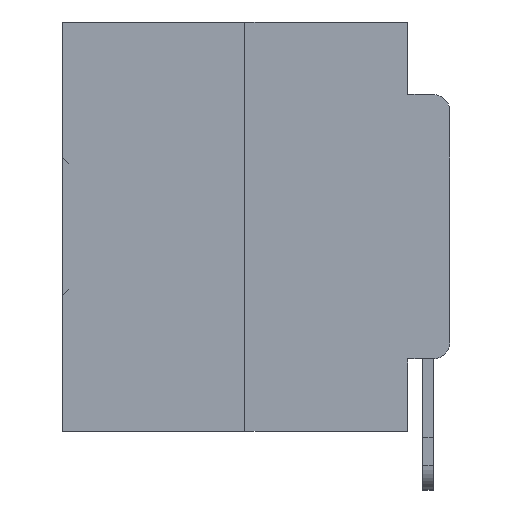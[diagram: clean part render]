
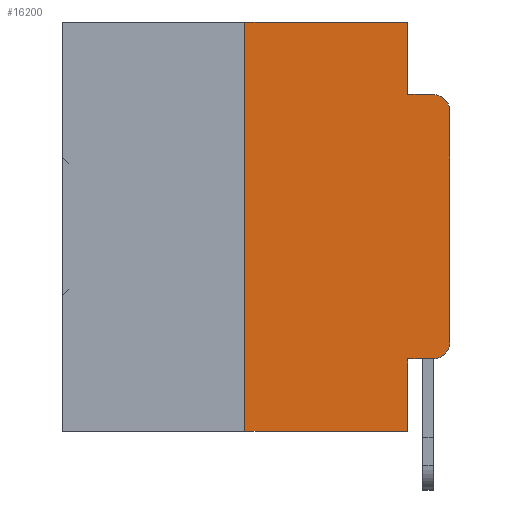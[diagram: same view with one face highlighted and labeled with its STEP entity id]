
A CAD part, left-side view. The second image highlights one B-rep face of the part: STEP entity #16200.
In plain terms, the highlighted planar face has unit normal (-1, 0, 0).
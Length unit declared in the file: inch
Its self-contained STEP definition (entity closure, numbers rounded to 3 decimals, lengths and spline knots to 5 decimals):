
#316 = ORIENTED_EDGE ( 'NONE', *, *, #16599, .T. ) ;
#415 = LINE ( 'NONE', #3776, #14605 ) ;
#475 = CARTESIAN_POINT ( 'NONE',  ( 0., 0.02, -0.1085 ) ) ;
#626 = AXIS2_PLACEMENT_3D ( 'NONE', #31320, #15009, #33985 ) ;
#838 = ORIENTED_EDGE ( 'NONE', *, *, #1508, .T. ) ;
#1125 = ORIENTED_EDGE ( 'NONE', *, *, #10313, .T. ) ;
#1165 = ORIENTED_EDGE ( 'NONE', *, *, #22442, .F. ) ;
#1508 = EDGE_CURVE ( 'NONE', #34756, #16977, #32853, .T. ) ;
#1520 = CARTESIAN_POINT ( 'NONE',  ( 0., 0.051, -0.4115 ) ) ;
#2182 = DIRECTION ( 'NONE',  ( 0., 0., -1. ) ) ;
#2471 = EDGE_CURVE ( 'NONE', #23822, #13464, #30337, .T. ) ;
#2742 = ORIENTED_EDGE ( 'NONE', *, *, #3702, .F. ) ;
#2930 = CARTESIAN_POINT ( 'NONE',  ( 0., 0.051, -0.4115 ) ) ;
#3365 = DIRECTION ( 'NONE',  ( 0., 0., -1. ) ) ;
#3394 = VERTEX_POINT ( 'NONE', #32758 ) ;
#3702 = EDGE_CURVE ( 'NONE', #13464, #31263, #34383, .T. ) ;
#3776 = CARTESIAN_POINT ( 'NONE',  ( 0., 0.051, 0. ) ) ;
#4247 = VECTOR ( 'NONE', #34108, 39.37008 ) ;
#5281 = EDGE_LOOP ( 'NONE', ( #1125, #838, #5604, #1165, #2742, #10926, #316, #14010, #35750, #34200 ) ) ;
#5604 = ORIENTED_EDGE ( 'NONE', *, *, #24743, .F. ) ;
#5786 = EDGE_CURVE ( 'NONE', #6816, #3394, #32164, .T. ) ;
#6456 = LINE ( 'NONE', #19384, #34750 ) ;
#6816 = VERTEX_POINT ( 'NONE', #9810 ) ;
#7062 = VECTOR ( 'NONE', #35310, 39.37008 ) ;
#7760 = CARTESIAN_POINT ( 'NONE',  ( 0., 0.051, 0. ) ) ;
#8363 = VECTOR ( 'NONE', #26809, 39.37008 ) ;
#8773 = LINE ( 'NONE', #1520, #22715 ) ;
#8868 = DIRECTION ( 'NONE',  ( 0., -1., 0. ) ) ;
#9810 = CARTESIAN_POINT ( 'NONE',  ( 0., 0.02, -0.4115 ) ) ;
#10313 = EDGE_CURVE ( 'NONE', #3394, #34756, #6456, .T. ) ;
#10926 = ORIENTED_EDGE ( 'NONE', *, *, #2471, .F. ) ;
#11040 = DIRECTION ( 'NONE',  ( 0., 0., 1. ) ) ;
#11996 = CARTESIAN_POINT ( 'NONE',  ( 0., 0., -0.1085 ) ) ;
#12901 = CARTESIAN_POINT ( 'NONE',  ( 0., 0.25, -0.5 ) ) ;
#13464 = VERTEX_POINT ( 'NONE', #29879 ) ;
#13774 = CARTESIAN_POINT ( 'NONE',  ( 0., 0.051, -0.5 ) ) ;
#14010 = ORIENTED_EDGE ( 'NONE', *, *, #14531, .F. ) ;
#14379 = VECTOR ( 'NONE', #8868, 39.37008 ) ;
#14531 = EDGE_CURVE ( 'NONE', #31238, #26175, #24023, .T. ) ;
#14605 = VECTOR ( 'NONE', #23334, 39.37008 ) ;
#15009 = DIRECTION ( 'NONE',  ( 1., 0., 0. ) ) ;
#15206 = EDGE_CURVE ( 'NONE', #31238, #6816, #8773, .T. ) ;
#15773 = CARTESIAN_POINT ( 'NONE',  ( 0., 0.25, 0. ) ) ;
#16200 = ADVANCED_FACE ( 'NONE', ( #27295 ), #33211, .F. ) ;
#16424 = CARTESIAN_POINT ( 'NONE',  ( 0., 0.051, -0.0885 ) ) ;
#16599 = EDGE_CURVE ( 'NONE', #23822, #26175, #21743, .T. ) ;
#16977 = VERTEX_POINT ( 'NONE', #21761 ) ;
#19093 = DIRECTION ( 'NONE',  ( -1., 0., 0. ) ) ;
#19384 = CARTESIAN_POINT ( 'NONE',  ( 0., 0., 0. ) ) ;
#19810 = VERTEX_POINT ( 'NONE', #34322 ) ;
#20209 = DIRECTION ( 'NONE',  ( -1., 0., 0. ) ) ;
#21052 = LINE ( 'NONE', #16424, #7062 ) ;
#21675 = DIRECTION ( 'NONE',  ( 0., 0., -1. ) ) ;
#21743 = LINE ( 'NONE', #25369, #14379 ) ;
#21761 = CARTESIAN_POINT ( 'NONE',  ( 0., 0.02, -0.0885 ) ) ;
#22442 = EDGE_CURVE ( 'NONE', #31263, #19810, #415, .T. ) ;
#22715 = VECTOR ( 'NONE', #26657, 39.37008 ) ;
#23334 = DIRECTION ( 'NONE',  ( 0., 0., -1. ) ) ;
#23822 = VERTEX_POINT ( 'NONE', #12901 ) ;
#24023 = LINE ( 'NONE', #7760, #29497 ) ;
#24743 = EDGE_CURVE ( 'NONE', #19810, #16977, #21052, .T. ) ;
#25369 = CARTESIAN_POINT ( 'NONE',  ( 0., 0.473, -0.5 ) ) ;
#25373 = CARTESIAN_POINT ( 'NONE',  ( 0., 0.051, 0. ) ) ;
#26175 = VERTEX_POINT ( 'NONE', #13774 ) ;
#26657 = DIRECTION ( 'NONE',  ( 0., -1., 0. ) ) ;
#26809 = DIRECTION ( 'NONE',  ( 0., 0., 1. ) ) ;
#27295 = FACE_OUTER_BOUND ( 'NONE', #5281, .T. ) ;
#29497 = VECTOR ( 'NONE', #21675, 39.37008 ) ;
#29879 = CARTESIAN_POINT ( 'NONE',  ( 0., 0.25, 0. ) ) ;
#30337 = LINE ( 'NONE', #15773, #8363 ) ;
#30368 = AXIS2_PLACEMENT_3D ( 'NONE', #475, #20209, #3365 ) ;
#31238 = VERTEX_POINT ( 'NONE', #2930 ) ;
#31263 = VERTEX_POINT ( 'NONE', #25373 ) ;
#31320 = CARTESIAN_POINT ( 'NONE',  ( 0., 0.473, 0. ) ) ;
#31446 = CARTESIAN_POINT ( 'NONE',  ( 0., 0.473, 0. ) ) ;
#32164 = CIRCLE ( 'NONE', #33503, 0.02 ) ;
#32758 = CARTESIAN_POINT ( 'NONE',  ( 0., 0., -0.3915 ) ) ;
#32853 = CIRCLE ( 'NONE', #30368, 0.02 ) ;
#33211 = PLANE ( 'NONE',  #626 ) ;
#33503 = AXIS2_PLACEMENT_3D ( 'NONE', #35167, #19093, #2182 ) ;
#33985 = DIRECTION ( 'NONE',  ( 0., 0., -1. ) ) ;
#34108 = DIRECTION ( 'NONE',  ( 0., -1., 0. ) ) ;
#34200 = ORIENTED_EDGE ( 'NONE', *, *, #5786, .T. ) ;
#34322 = CARTESIAN_POINT ( 'NONE',  ( 0., 0.051, -0.0885 ) ) ;
#34383 = LINE ( 'NONE', #31446, #4247 ) ;
#34750 = VECTOR ( 'NONE', #11040, 39.37008 ) ;
#34756 = VERTEX_POINT ( 'NONE', #11996 ) ;
#35167 = CARTESIAN_POINT ( 'NONE',  ( 0., 0.02, -0.3915 ) ) ;
#35310 = DIRECTION ( 'NONE',  ( 0., -1., 0. ) ) ;
#35750 = ORIENTED_EDGE ( 'NONE', *, *, #15206, .T. ) ;
